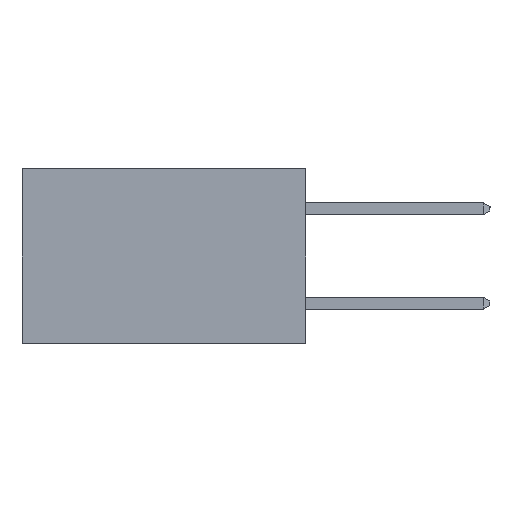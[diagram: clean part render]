
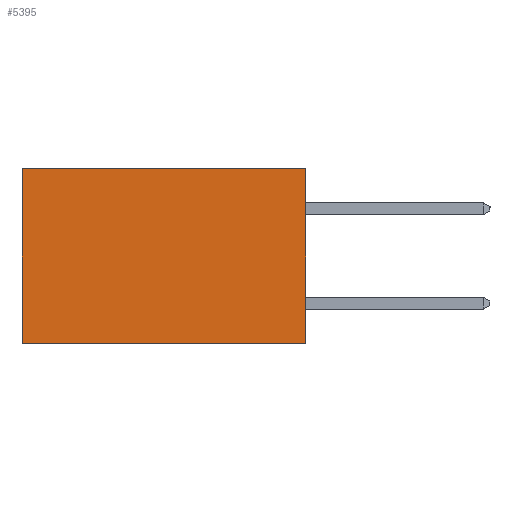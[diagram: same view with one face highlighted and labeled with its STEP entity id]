
A CAD part, left-side view. The second image highlights one B-rep face of the part: STEP entity #5395.
In plain terms, the highlighted planar face has unit normal (-1, 0, 0).
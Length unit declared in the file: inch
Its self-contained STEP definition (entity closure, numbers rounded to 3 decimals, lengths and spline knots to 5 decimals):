
#365 = VECTOR ( 'NONE', #6870, 39.37008 ) ;
#698 = VECTOR ( 'NONE', #7470, 39.37008 ) ;
#931 = AXIS2_PLACEMENT_3D ( 'NONE', #11606, #3403, #9796 ) ;
#1163 = EDGE_CURVE ( 'NONE', #10049, #12565, #17415, .T. ) ;
#1206 = CARTESIAN_POINT ( 'NONE',  ( 0.2615, 0., 0. ) ) ;
#1220 = EDGE_CURVE ( 'NONE', #12565, #18551, #9090, .T. ) ;
#2048 = CARTESIAN_POINT ( 'NONE',  ( 0.2615, 0., -0.37 ) ) ;
#2278 = CARTESIAN_POINT ( 'NONE',  ( 0.2615, 0., -0.37 ) ) ;
#2799 = CARTESIAN_POINT ( 'NONE',  ( 0.2615, 0.6, -0.37 ) ) ;
#3306 = FACE_OUTER_BOUND ( 'NONE', #14032, .T. ) ;
#3403 = DIRECTION ( 'NONE',  ( 1., 0., 0. ) ) ;
#3988 = DIRECTION ( 'NONE',  ( 0., 1., 0. ) ) ;
#5090 = PLANE ( 'NONE',  #931 ) ;
#5395 = ADVANCED_FACE ( 'NONE', ( #3306 ), #5090, .F. ) ;
#5665 = ORIENTED_EDGE ( 'NONE', *, *, #11898, .F. ) ;
#5757 = ORIENTED_EDGE ( 'NONE', *, *, #9743, .F. ) ;
#6393 = CARTESIAN_POINT ( 'NONE',  ( 0.2615, 0.6, -0.37 ) ) ;
#6870 = DIRECTION ( 'NONE',  ( 0., 0., -1. ) ) ;
#7470 = DIRECTION ( 'NONE',  ( 0., 0., -1. ) ) ;
#8683 = LINE ( 'NONE', #2278, #16814 ) ;
#9090 = LINE ( 'NONE', #2799, #698 ) ;
#9743 = EDGE_CURVE ( 'NONE', #10049, #19481, #13384, .T. ) ;
#9796 = DIRECTION ( 'NONE',  ( 0., 0., -1. ) ) ;
#9822 = ORIENTED_EDGE ( 'NONE', *, *, #1163, .T. ) ;
#10049 = VERTEX_POINT ( 'NONE', #1206 ) ;
#10566 = DIRECTION ( 'NONE',  ( 0., 1., 0. ) ) ;
#10756 = CARTESIAN_POINT ( 'NONE',  ( 0.2615, 0.6, 0. ) ) ;
#10789 = CARTESIAN_POINT ( 'NONE',  ( 0.2615, 0., 0. ) ) ;
#11606 = CARTESIAN_POINT ( 'NONE',  ( 0.2615, 0., -0.37 ) ) ;
#11898 = EDGE_CURVE ( 'NONE', #19481, #18551, #8683, .T. ) ;
#12042 = VECTOR ( 'NONE', #10566, 39.37008 ) ;
#12565 = VERTEX_POINT ( 'NONE', #10756 ) ;
#13384 = LINE ( 'NONE', #18306, #365 ) ;
#14032 = EDGE_LOOP ( 'NONE', ( #20256, #5665, #5757, #9822 ) ) ;
#16814 = VECTOR ( 'NONE', #3988, 39.37008 ) ;
#17415 = LINE ( 'NONE', #10789, #12042 ) ;
#18306 = CARTESIAN_POINT ( 'NONE',  ( 0.2615, 0., -0.37 ) ) ;
#18551 = VERTEX_POINT ( 'NONE', #6393 ) ;
#19481 = VERTEX_POINT ( 'NONE', #2048 ) ;
#20256 = ORIENTED_EDGE ( 'NONE', *, *, #1220, .T. ) ;
